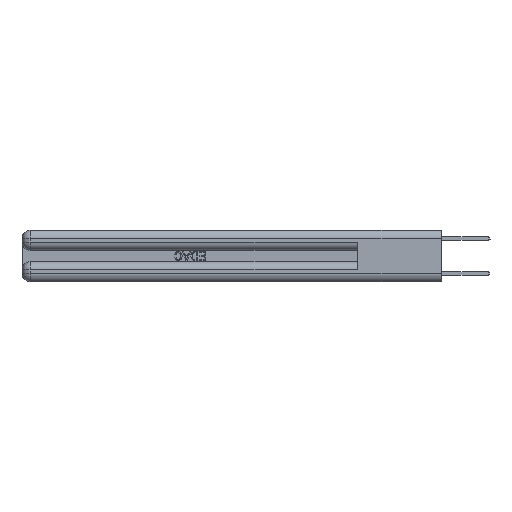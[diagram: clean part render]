
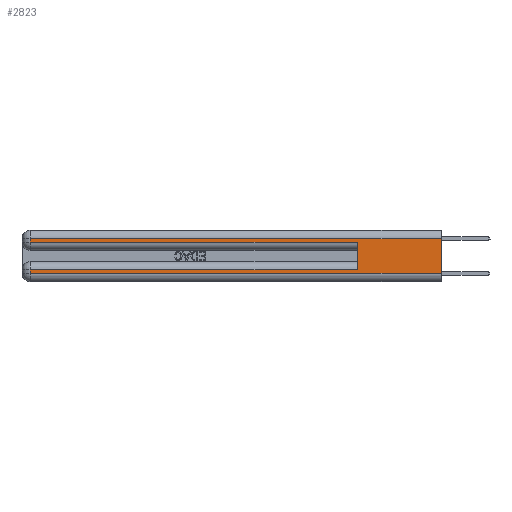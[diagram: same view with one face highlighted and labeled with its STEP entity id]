
A CAD part, left-side view. The second image highlights one B-rep face of the part: STEP entity #2823.
In plain terms, the highlighted planar face has unit normal (-1, 0, 0).
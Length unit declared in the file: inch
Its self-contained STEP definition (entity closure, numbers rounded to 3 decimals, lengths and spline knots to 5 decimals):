
#299 = LINE ( 'NONE', #15640, #20891 ) ;
#1275 = EDGE_CURVE ( 'NONE', #9666, #4053, #299, .T. ) ;
#1435 = VERTEX_POINT ( 'NONE', #23855 ) ;
#1829 = DIRECTION ( 'NONE',  ( 0., 1., 0. ) ) ;
#1834 = VERTEX_POINT ( 'NONE', #25759 ) ;
#2823 = ADVANCED_FACE ( 'NONE', ( #8257 ), #11201, .F. ) ;
#3132 = CARTESIAN_POINT ( 'NONE',  ( 0., 2.94, 0.285 ) ) ;
#3348 = CARTESIAN_POINT ( 'NONE',  ( 0., 0., 0.285 ) ) ;
#3855 = VECTOR ( 'NONE', #1829, 39.37008 ) ;
#4053 = VERTEX_POINT ( 'NONE', #21400 ) ;
#5068 = LINE ( 'NONE', #6662, #23786 ) ;
#5809 = DIRECTION ( 'NONE',  ( 0., -1., 0. ) ) ;
#6636 = VERTEX_POINT ( 'NONE', #25368 ) ;
#6662 = CARTESIAN_POINT ( 'NONE',  ( 0., 2.94, 0.37 ) ) ;
#7674 = EDGE_CURVE ( 'NONE', #1834, #1435, #19893, .T. ) ;
#8257 = FACE_OUTER_BOUND ( 'NONE', #16108, .T. ) ;
#9666 = VERTEX_POINT ( 'NONE', #14775 ) ;
#9786 = ORIENTED_EDGE ( 'NONE', *, *, #22637, .T. ) ;
#10832 = ORIENTED_EDGE ( 'NONE', *, *, #1275, .T. ) ;
#11072 = LINE ( 'NONE', #22349, #29844 ) ;
#11201 = PLANE ( 'NONE',  #22029 ) ;
#11306 = DIRECTION ( 'NONE',  ( 1., 0., 0. ) ) ;
#12381 = LINE ( 'NONE', #30750, #27323 ) ;
#12386 = DIRECTION ( 'NONE',  ( 0., 0., 1. ) ) ;
#12411 = EDGE_CURVE ( 'NONE', #1834, #18696, #26065, .T. ) ;
#13368 = DIRECTION ( 'NONE',  ( 0., 0., -1. ) ) ;
#13422 = VECTOR ( 'NONE', #19668, 39.37008 ) ;
#13664 = CARTESIAN_POINT ( 'NONE',  ( 0., 0.6, 0.285 ) ) ;
#14733 = ORIENTED_EDGE ( 'NONE', *, *, #30908, .F. ) ;
#14775 = CARTESIAN_POINT ( 'NONE',  ( 0., 2.94, 0.085 ) ) ;
#15274 = CARTESIAN_POINT ( 'NONE',  ( 0., 0., 0.085 ) ) ;
#15640 = CARTESIAN_POINT ( 'NONE',  ( 0., 2.94, 0.37 ) ) ;
#16108 = EDGE_LOOP ( 'NONE', ( #22279, #18207, #9786, #18483, #14733, #20467, #10832, #20853 ) ) ;
#16544 = CARTESIAN_POINT ( 'NONE',  ( 0., 0., 0.37 ) ) ;
#16553 = DIRECTION ( 'NONE',  ( 0., 0., -1. ) ) ;
#17576 = VECTOR ( 'NONE', #5809, 39.37008 ) ;
#18207 = ORIENTED_EDGE ( 'NONE', *, *, #7674, .T. ) ;
#18483 = ORIENTED_EDGE ( 'NONE', *, *, #31201, .T. ) ;
#18509 = DIRECTION ( 'NONE',  ( 0., 0., -1. ) ) ;
#18696 = VERTEX_POINT ( 'NONE', #22445 ) ;
#19668 = DIRECTION ( 'NONE',  ( 0., 1., 0. ) ) ;
#19893 = LINE ( 'NONE', #23924, #3855 ) ;
#19960 = LINE ( 'NONE', #15274, #13422 ) ;
#20467 = ORIENTED_EDGE ( 'NONE', *, *, #29335, .T. ) ;
#20853 = ORIENTED_EDGE ( 'NONE', *, *, #27882, .T. ) ;
#20891 = VECTOR ( 'NONE', #13368, 39.37008 ) ;
#21029 = DIRECTION ( 'NONE',  ( 0., 0., -1. ) ) ;
#21225 = DIRECTION ( 'NONE',  ( 0., -1., 0. ) ) ;
#21400 = CARTESIAN_POINT ( 'NONE',  ( 0., 2.94, 0.06 ) ) ;
#22029 = AXIS2_PLACEMENT_3D ( 'NONE', #23515, #11306, #16553 ) ;
#22279 = ORIENTED_EDGE ( 'NONE', *, *, #12411, .F. ) ;
#22349 = CARTESIAN_POINT ( 'NONE',  ( 0., 0.6, 0.145 ) ) ;
#22445 = CARTESIAN_POINT ( 'NONE',  ( 0., 0., 0.06 ) ) ;
#22637 = EDGE_CURVE ( 'NONE', #1435, #31134, #5068, .T. ) ;
#23515 = CARTESIAN_POINT ( 'NONE',  ( 0., 0., 0.37 ) ) ;
#23786 = VECTOR ( 'NONE', #18509, 39.37008 ) ;
#23855 = CARTESIAN_POINT ( 'NONE',  ( 0., 2.94, 0.31 ) ) ;
#23924 = CARTESIAN_POINT ( 'NONE',  ( 0., 0., 0.31 ) ) ;
#25368 = CARTESIAN_POINT ( 'NONE',  ( 0., 0.6, 0.085 ) ) ;
#25759 = CARTESIAN_POINT ( 'NONE',  ( 0., 0., 0.31 ) ) ;
#26065 = LINE ( 'NONE', #16544, #30270 ) ;
#26379 = LINE ( 'NONE', #3348, #17576 ) ;
#27115 = VERTEX_POINT ( 'NONE', #13664 ) ;
#27323 = VECTOR ( 'NONE', #21225, 39.37008 ) ;
#27882 = EDGE_CURVE ( 'NONE', #4053, #18696, #12381, .T. ) ;
#29335 = EDGE_CURVE ( 'NONE', #6636, #9666, #19960, .T. ) ;
#29844 = VECTOR ( 'NONE', #12386, 39.37008 ) ;
#30270 = VECTOR ( 'NONE', #21029, 39.37008 ) ;
#30750 = CARTESIAN_POINT ( 'NONE',  ( 0., 0., 0.06 ) ) ;
#30908 = EDGE_CURVE ( 'NONE', #6636, #27115, #11072, .T. ) ;
#31134 = VERTEX_POINT ( 'NONE', #3132 ) ;
#31201 = EDGE_CURVE ( 'NONE', #31134, #27115, #26379, .T. ) ;
